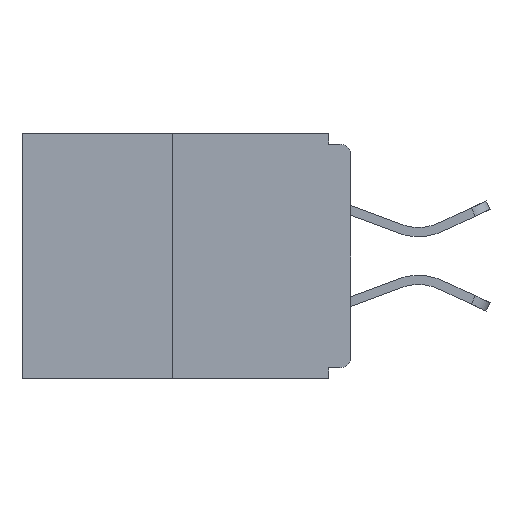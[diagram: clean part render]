
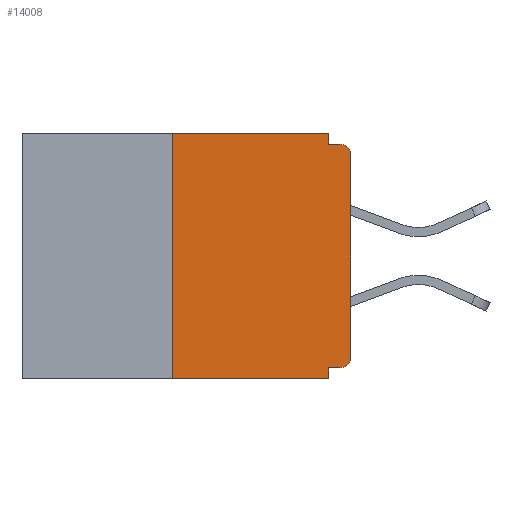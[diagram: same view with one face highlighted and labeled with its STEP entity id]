
A CAD part, left-side view. The second image highlights one B-rep face of the part: STEP entity #14008.
In plain terms, the highlighted planar face has unit normal (-1, 0, 0).
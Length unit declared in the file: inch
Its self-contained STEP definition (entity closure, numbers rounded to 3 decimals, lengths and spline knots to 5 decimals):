
#635 = DIRECTION ( 'NONE',  ( -1., 0., 0. ) ) ;
#738 = ORIENTED_EDGE ( 'NONE', *, *, #12595, .F. ) ;
#893 = LINE ( 'NONE', #3659, #10663 ) ;
#1440 = VERTEX_POINT ( 'NONE', #20176 ) ;
#1588 = EDGE_CURVE ( 'NONE', #2815, #20319, #6568, .T. ) ;
#1862 = EDGE_CURVE ( 'NONE', #2815, #7248, #6824, .T. ) ;
#1934 = ORIENTED_EDGE ( 'NONE', *, *, #7268, .F. ) ;
#2097 = VECTOR ( 'NONE', #4662, 39.37008 ) ;
#2327 = LINE ( 'NONE', #21194, #6764 ) ;
#2332 = VERTEX_POINT ( 'NONE', #15081 ) ;
#2815 = VERTEX_POINT ( 'NONE', #17768 ) ;
#3028 = CARTESIAN_POINT ( 'NONE',  ( 0., 0., -0.328 ) ) ;
#3233 = CARTESIAN_POINT ( 'NONE',  ( 0., 0.031, -0.343 ) ) ;
#3538 = CARTESIAN_POINT ( 'NONE',  ( 0., 0.031, -0.328 ) ) ;
#3659 = CARTESIAN_POINT ( 'NONE',  ( 0., 0.46, 0. ) ) ;
#4018 = CARTESIAN_POINT ( 'NONE',  ( 0., 0., -0.313 ) ) ;
#4364 = DIRECTION ( 'NONE',  ( 0., 0., -1. ) ) ;
#4662 = DIRECTION ( 'NONE',  ( 0., 1., 0. ) ) ;
#4735 = VECTOR ( 'NONE', #14108, 39.37008 ) ;
#4922 = ORIENTED_EDGE ( 'NONE', *, *, #16428, .T. ) ;
#4959 = CARTESIAN_POINT ( 'NONE',  ( 0., 0.031, 0. ) ) ;
#5366 = CIRCLE ( 'NONE', #9510, 0.015 ) ;
#5810 = EDGE_CURVE ( 'NONE', #6679, #2332, #5366, .T. ) ;
#6012 = ORIENTED_EDGE ( 'NONE', *, *, #16302, .F. ) ;
#6075 = CARTESIAN_POINT ( 'NONE',  ( 0., 0.015, -0.03 ) ) ;
#6543 = CARTESIAN_POINT ( 'NONE',  ( 0., 0.015, -0.313 ) ) ;
#6568 = CIRCLE ( 'NONE', #14216, 0.015 ) ;
#6679 = VERTEX_POINT ( 'NONE', #17033 ) ;
#6764 = VECTOR ( 'NONE', #10686, 39.37008 ) ;
#6824 = LINE ( 'NONE', #3028, #2097 ) ;
#7248 = VERTEX_POINT ( 'NONE', #3538 ) ;
#7268 = EDGE_CURVE ( 'NONE', #7248, #11085, #2327, .T. ) ;
#8486 = PLANE ( 'NONE',  #11472 ) ;
#8554 = DIRECTION ( 'NONE',  ( 0., 0., -1. ) ) ;
#8691 = VECTOR ( 'NONE', #16707, 39.37008 ) ;
#8838 = LINE ( 'NONE', #16695, #21630 ) ;
#8900 = CARTESIAN_POINT ( 'NONE',  ( 0., 0.25, 0. ) ) ;
#9349 = DIRECTION ( 'NONE',  ( 0., 0., -1. ) ) ;
#9510 = AXIS2_PLACEMENT_3D ( 'NONE', #6075, #635, #9349 ) ;
#9796 = CARTESIAN_POINT ( 'NONE',  ( 0., 0.46, 0. ) ) ;
#9856 = DIRECTION ( 'NONE',  ( 1., 0., 0. ) ) ;
#9981 = FACE_OUTER_BOUND ( 'NONE', #16224, .T. ) ;
#10002 = LINE ( 'NONE', #8900, #4735 ) ;
#10512 = ORIENTED_EDGE ( 'NONE', *, *, #13793, .F. ) ;
#10625 = VECTOR ( 'NONE', #13172, 39.37008 ) ;
#10663 = VECTOR ( 'NONE', #17717, 39.37008 ) ;
#10686 = DIRECTION ( 'NONE',  ( 0., 0., -1. ) ) ;
#11085 = VERTEX_POINT ( 'NONE', #3233 ) ;
#11472 = AXIS2_PLACEMENT_3D ( 'NONE', #9796, #9856, #4364 ) ;
#11622 = ORIENTED_EDGE ( 'NONE', *, *, #1588, .T. ) ;
#12042 = CARTESIAN_POINT ( 'NONE',  ( 0., 0.031, 0. ) ) ;
#12595 = EDGE_CURVE ( 'NONE', #1440, #17134, #10002, .T. ) ;
#12798 = CARTESIAN_POINT ( 'NONE',  ( 0., 0., -0.015 ) ) ;
#13172 = DIRECTION ( 'NONE',  ( 0., -1., 0. ) ) ;
#13793 = EDGE_CURVE ( 'NONE', #14212, #18718, #18079, .T. ) ;
#13975 = LINE ( 'NONE', #12798, #8691 ) ;
#14008 = ADVANCED_FACE ( 'NONE', ( #9981 ), #8486, .F. ) ;
#14108 = DIRECTION ( 'NONE',  ( 0., 0., 1. ) ) ;
#14212 = VERTEX_POINT ( 'NONE', #4959 ) ;
#14216 = AXIS2_PLACEMENT_3D ( 'NONE', #6543, #17426, #21084 ) ;
#14654 = EDGE_CURVE ( 'NONE', #20319, #6679, #8838, .T. ) ;
#14761 = CARTESIAN_POINT ( 'NONE',  ( 0., 0.46, -0.343 ) ) ;
#15081 = CARTESIAN_POINT ( 'NONE',  ( 0., 0.015, -0.015 ) ) ;
#15595 = CARTESIAN_POINT ( 'NONE',  ( 0., 0.031, -0.015 ) ) ;
#15787 = ORIENTED_EDGE ( 'NONE', *, *, #5810, .T. ) ;
#15854 = VECTOR ( 'NONE', #8554, 39.37008 ) ;
#16224 = EDGE_LOOP ( 'NONE', ( #21013, #738, #4922, #1934, #19732, #11622, #16928, #15787, #6012, #10512 ) ) ;
#16302 = EDGE_CURVE ( 'NONE', #18718, #2332, #13975, .T. ) ;
#16428 = EDGE_CURVE ( 'NONE', #1440, #11085, #20108, .T. ) ;
#16695 = CARTESIAN_POINT ( 'NONE',  ( 0., 0., 0. ) ) ;
#16707 = DIRECTION ( 'NONE',  ( 0., -1., 0. ) ) ;
#16928 = ORIENTED_EDGE ( 'NONE', *, *, #14654, .T. ) ;
#17021 = CARTESIAN_POINT ( 'NONE',  ( 0., 0.25, 0. ) ) ;
#17033 = CARTESIAN_POINT ( 'NONE',  ( 0., 0., -0.03 ) ) ;
#17134 = VERTEX_POINT ( 'NONE', #17021 ) ;
#17426 = DIRECTION ( 'NONE',  ( -1., 0., 0. ) ) ;
#17717 = DIRECTION ( 'NONE',  ( 0., -1., 0. ) ) ;
#17768 = CARTESIAN_POINT ( 'NONE',  ( 0., 0.015, -0.328 ) ) ;
#18079 = LINE ( 'NONE', #12042, #15854 ) ;
#18718 = VERTEX_POINT ( 'NONE', #15595 ) ;
#19732 = ORIENTED_EDGE ( 'NONE', *, *, #1862, .F. ) ;
#20108 = LINE ( 'NONE', #14761, #10625 ) ;
#20129 = DIRECTION ( 'NONE',  ( 0., 0., 1. ) ) ;
#20176 = CARTESIAN_POINT ( 'NONE',  ( 0., 0.25, -0.343 ) ) ;
#20319 = VERTEX_POINT ( 'NONE', #4018 ) ;
#21013 = ORIENTED_EDGE ( 'NONE', *, *, #21751, .F. ) ;
#21084 = DIRECTION ( 'NONE',  ( 0., 0., -1. ) ) ;
#21194 = CARTESIAN_POINT ( 'NONE',  ( 0., 0.031, -0.343 ) ) ;
#21630 = VECTOR ( 'NONE', #20129, 39.37008 ) ;
#21751 = EDGE_CURVE ( 'NONE', #17134, #14212, #893, .T. ) ;
